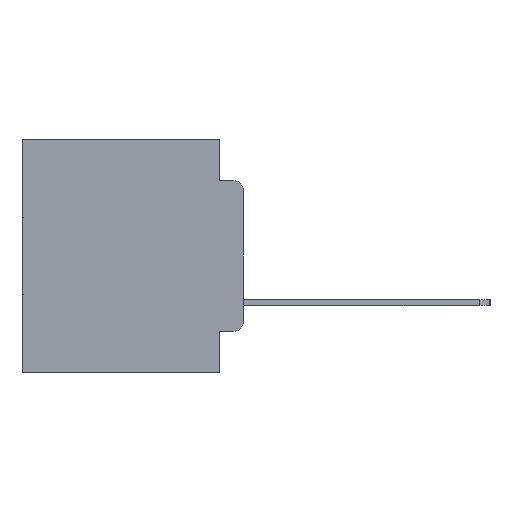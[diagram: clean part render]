
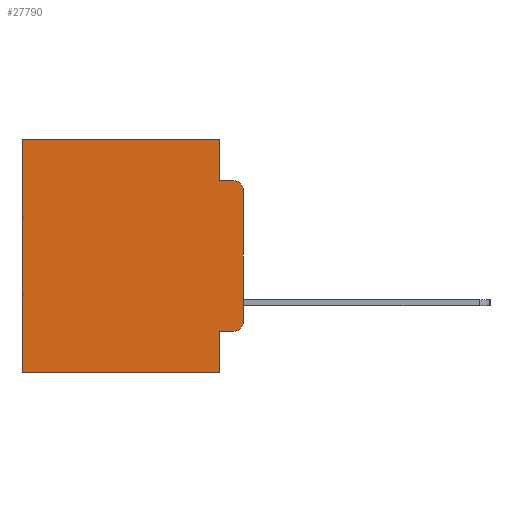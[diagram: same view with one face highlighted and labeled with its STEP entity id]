
A CAD part, left-side view. The second image highlights one B-rep face of the part: STEP entity #27790.
In plain terms, the highlighted planar face has unit normal (-1, 0, 0).
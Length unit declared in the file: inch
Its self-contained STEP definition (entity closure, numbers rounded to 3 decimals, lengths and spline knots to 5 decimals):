
#111 = ORIENTED_EDGE ( 'NONE', *, *, #20865, .F. ) ;
#371 = LINE ( 'NONE', #28492, #18892 ) ;
#427 = CARTESIAN_POINT ( 'NONE',  ( 0.298, 0.02, -0.4115 ) ) ;
#473 = EDGE_CURVE ( 'NONE', #9546, #5722, #20392, .T. ) ;
#798 = CARTESIAN_POINT ( 'NONE',  ( 0.298, 0.051, -0.4115 ) ) ;
#1008 = VERTEX_POINT ( 'NONE', #17373 ) ;
#1031 = AXIS2_PLACEMENT_3D ( 'NONE', #22593, #8277, #24951 ) ;
#1697 = AXIS2_PLACEMENT_3D ( 'NONE', #4271, #21062, #6703 ) ;
#2244 = VERTEX_POINT ( 'NONE', #28714 ) ;
#2903 = DIRECTION ( 'NONE',  ( 0., -1., 0. ) ) ;
#3555 = CIRCLE ( 'NONE', #1697, 0.02 ) ;
#4271 = CARTESIAN_POINT ( 'NONE',  ( 0.298, 0.02, -0.3915 ) ) ;
#4359 = EDGE_CURVE ( 'NONE', #6021, #26133, #24778, .T. ) ;
#4991 = LINE ( 'NONE', #20609, #10676 ) ;
#5722 = VERTEX_POINT ( 'NONE', #427 ) ;
#6021 = VERTEX_POINT ( 'NONE', #8882 ) ;
#6084 = VECTOR ( 'NONE', #26965, 39.37008 ) ;
#6358 = CARTESIAN_POINT ( 'NONE',  ( 0.298, 0.473, 0. ) ) ;
#6597 = VECTOR ( 'NONE', #29999, 39.37008 ) ;
#6703 = DIRECTION ( 'NONE',  ( 0., 0., -1. ) ) ;
#6996 = ORIENTED_EDGE ( 'NONE', *, *, #23496, .T. ) ;
#7062 = ORIENTED_EDGE ( 'NONE', *, *, #11488, .T. ) ;
#8230 = EDGE_LOOP ( 'NONE', ( #10400, #6996, #20499, #13750, #30828, #10113, #14899, #111, #20911, #7062 ) ) ;
#8277 = DIRECTION ( 'NONE',  ( -1., 0., 0. ) ) ;
#8684 = DIRECTION ( 'NONE',  ( 0., 0., -1. ) ) ;
#8688 = EDGE_CURVE ( 'NONE', #30207, #1008, #8897, .T. ) ;
#8882 = CARTESIAN_POINT ( 'NONE',  ( 0.298, 0., -0.1085 ) ) ;
#8897 = LINE ( 'NONE', #6358, #14485 ) ;
#9546 = VERTEX_POINT ( 'NONE', #798 ) ;
#10113 = ORIENTED_EDGE ( 'NONE', *, *, #8688, .T. ) ;
#10152 = VERTEX_POINT ( 'NONE', #15262 ) ;
#10165 = CARTESIAN_POINT ( 'NONE',  ( 0.298, 0., -0.5 ) ) ;
#10253 = EDGE_CURVE ( 'NONE', #26868, #30207, #20863, .T. ) ;
#10400 = ORIENTED_EDGE ( 'NONE', *, *, #4359, .F. ) ;
#10676 = VECTOR ( 'NONE', #8684, 39.37008 ) ;
#11488 = EDGE_CURVE ( 'NONE', #5722, #26133, #3555, .T. ) ;
#11657 = CARTESIAN_POINT ( 'NONE',  ( 0.298, 0.051, -0.4115 ) ) ;
#12091 = AXIS2_PLACEMENT_3D ( 'NONE', #12698, #12797, #29413 ) ;
#12698 = CARTESIAN_POINT ( 'NONE',  ( 0.298, 0., 0. ) ) ;
#12797 = DIRECTION ( 'NONE',  ( 1., 0., 0. ) ) ;
#13750 = ORIENTED_EDGE ( 'NONE', *, *, #28192, .F. ) ;
#14000 = VECTOR ( 'NONE', #2903, 39.37008 ) ;
#14232 = DIRECTION ( 'NONE',  ( 0., 0., -1. ) ) ;
#14485 = VECTOR ( 'NONE', #25483, 39.37008 ) ;
#14826 = DIRECTION ( 'NONE',  ( 0., 1., 0. ) ) ;
#14899 = ORIENTED_EDGE ( 'NONE', *, *, #19363, .F. ) ;
#15262 = CARTESIAN_POINT ( 'NONE',  ( 0.298, 0.051, -0.5 ) ) ;
#17373 = CARTESIAN_POINT ( 'NONE',  ( 0.298, 0.473, -0.5 ) ) ;
#17800 = LINE ( 'NONE', #10165, #24131 ) ;
#18892 = VECTOR ( 'NONE', #14232, 39.37008 ) ;
#19363 = EDGE_CURVE ( 'NONE', #10152, #1008, #17800, .T. ) ;
#19933 = PLANE ( 'NONE',  #12091 ) ;
#20392 = LINE ( 'NONE', #11657, #14000 ) ;
#20499 = ORIENTED_EDGE ( 'NONE', *, *, #29022, .F. ) ;
#20609 = CARTESIAN_POINT ( 'NONE',  ( 0.298, 0.051, 0. ) ) ;
#20863 = LINE ( 'NONE', #27638, #6597 ) ;
#20865 = EDGE_CURVE ( 'NONE', #9546, #10152, #4991, .T. ) ;
#20911 = ORIENTED_EDGE ( 'NONE', *, *, #473, .T. ) ;
#21062 = DIRECTION ( 'NONE',  ( -1., 0., 0. ) ) ;
#22593 = CARTESIAN_POINT ( 'NONE',  ( 0.298, 0.02, -0.1085 ) ) ;
#23486 = CARTESIAN_POINT ( 'NONE',  ( 0.298, 0., -0.3915 ) ) ;
#23496 = EDGE_CURVE ( 'NONE', #6021, #2244, #27337, .T. ) ;
#23570 = CARTESIAN_POINT ( 'NONE',  ( 0.298, 0., 0. ) ) ;
#24044 = VERTEX_POINT ( 'NONE', #26989 ) ;
#24131 = VECTOR ( 'NONE', #14826, 39.37008 ) ;
#24693 = CARTESIAN_POINT ( 'NONE',  ( 0.298, 0.051, -0.0885 ) ) ;
#24778 = LINE ( 'NONE', #23570, #30298 ) ;
#24951 = DIRECTION ( 'NONE',  ( 0., 0., -1. ) ) ;
#25483 = DIRECTION ( 'NONE',  ( 0., 0., -1. ) ) ;
#25552 = CARTESIAN_POINT ( 'NONE',  ( 0.298, 0.051, 0. ) ) ;
#25554 = CARTESIAN_POINT ( 'NONE',  ( 0.298, 0.473, 0. ) ) ;
#26133 = VERTEX_POINT ( 'NONE', #23486 ) ;
#26868 = VERTEX_POINT ( 'NONE', #25552 ) ;
#26965 = DIRECTION ( 'NONE',  ( 0., -1., 0. ) ) ;
#26989 = CARTESIAN_POINT ( 'NONE',  ( 0.298, 0.051, -0.0885 ) ) ;
#27337 = CIRCLE ( 'NONE', #1031, 0.02 ) ;
#27638 = CARTESIAN_POINT ( 'NONE',  ( 0.298, 0., 0. ) ) ;
#27790 = ADVANCED_FACE ( 'NONE', ( #30745 ), #19933, .F. ) ;
#28192 = EDGE_CURVE ( 'NONE', #26868, #24044, #371, .T. ) ;
#28323 = DIRECTION ( 'NONE',  ( 0., 0., -1. ) ) ;
#28492 = CARTESIAN_POINT ( 'NONE',  ( 0.298, 0.051, 0. ) ) ;
#28714 = CARTESIAN_POINT ( 'NONE',  ( 0.298, 0.02, -0.0885 ) ) ;
#29022 = EDGE_CURVE ( 'NONE', #24044, #2244, #30657, .T. ) ;
#29413 = DIRECTION ( 'NONE',  ( 0., 0., -1. ) ) ;
#29999 = DIRECTION ( 'NONE',  ( 0., 1., 0. ) ) ;
#30207 = VERTEX_POINT ( 'NONE', #25554 ) ;
#30298 = VECTOR ( 'NONE', #28323, 39.37008 ) ;
#30657 = LINE ( 'NONE', #24693, #6084 ) ;
#30745 = FACE_OUTER_BOUND ( 'NONE', #8230, .T. ) ;
#30828 = ORIENTED_EDGE ( 'NONE', *, *, #10253, .T. ) ;
